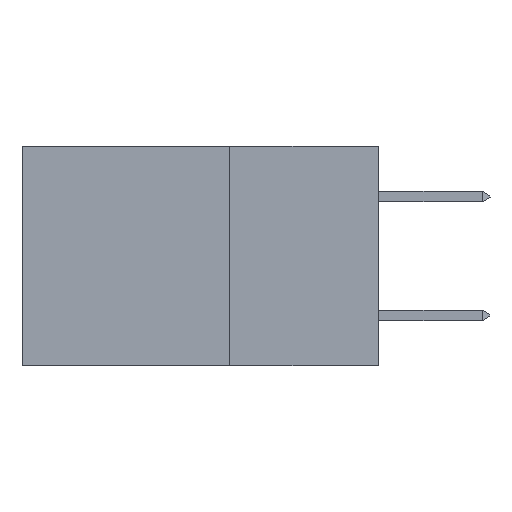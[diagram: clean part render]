
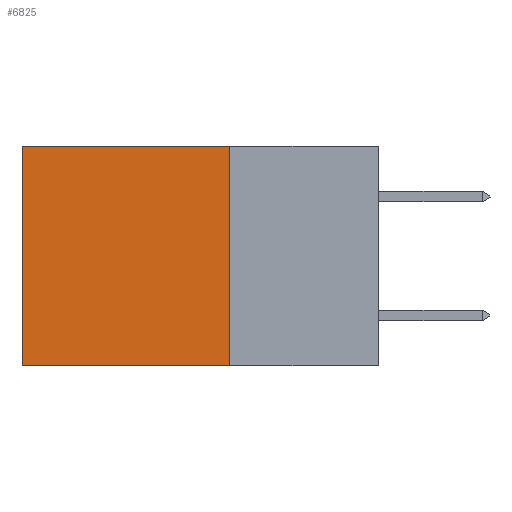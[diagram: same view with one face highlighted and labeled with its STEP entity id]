
A CAD part, left-side view. The second image highlights one B-rep face of the part: STEP entity #6825.
In plain terms, the highlighted planar face has unit normal (-1, 0, 0).
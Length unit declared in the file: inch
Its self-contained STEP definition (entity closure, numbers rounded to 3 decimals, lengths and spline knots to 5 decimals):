
#5 = VERTEX_POINT ( 'NONE', #8557 ) ;
#57 = VECTOR ( 'NONE', #5633, 39.37008 ) ;
#301 = CARTESIAN_POINT ( 'NONE',  ( 0.298, 0.25, -0.37 ) ) ;
#320 = EDGE_CURVE ( 'NONE', #5, #7598, #5847, .T. ) ;
#431 = EDGE_LOOP ( 'NONE', ( #5584, #6023, #5073, #2208 ) ) ;
#1246 = DIRECTION ( 'NONE',  ( 0., 1., 0. ) ) ;
#1287 = EDGE_CURVE ( 'NONE', #1420, #7598, #6776, .T. ) ;
#1373 = AXIS2_PLACEMENT_3D ( 'NONE', #1584, #4476, #4543 ) ;
#1420 = VERTEX_POINT ( 'NONE', #301 ) ;
#1573 = CARTESIAN_POINT ( 'NONE',  ( 0.298, 0.25, -0.37 ) ) ;
#1584 = CARTESIAN_POINT ( 'NONE',  ( 0.298, 0.25, 0. ) ) ;
#1973 = CARTESIAN_POINT ( 'NONE',  ( 0.298, 0.6, 0. ) ) ;
#2208 = ORIENTED_EDGE ( 'NONE', *, *, #9038, .T. ) ;
#2286 = LINE ( 'NONE', #8377, #9173 ) ;
#2630 = LINE ( 'NONE', #6064, #7817 ) ;
#3183 = EDGE_CURVE ( 'NONE', #4567, #1420, #2630, .T. ) ;
#4395 = FACE_OUTER_BOUND ( 'NONE', #431, .T. ) ;
#4476 = DIRECTION ( 'NONE',  ( 1., 0., 0. ) ) ;
#4543 = DIRECTION ( 'NONE',  ( 0., 0., -1. ) ) ;
#4567 = VERTEX_POINT ( 'NONE', #8984 ) ;
#4875 = CARTESIAN_POINT ( 'NONE',  ( 0.298, 0.6, -0.37 ) ) ;
#5073 = ORIENTED_EDGE ( 'NONE', *, *, #3183, .F. ) ;
#5584 = ORIENTED_EDGE ( 'NONE', *, *, #320, .T. ) ;
#5633 = DIRECTION ( 'NONE',  ( 0., 0., -1. ) ) ;
#5847 = LINE ( 'NONE', #1973, #57 ) ;
#6023 = ORIENTED_EDGE ( 'NONE', *, *, #1287, .F. ) ;
#6064 = CARTESIAN_POINT ( 'NONE',  ( 0.298, 0.25, 0. ) ) ;
#6776 = LINE ( 'NONE', #1573, #6995 ) ;
#6825 = ADVANCED_FACE ( 'NONE', ( #4395 ), #8909, .F. ) ;
#6995 = VECTOR ( 'NONE', #8244, 39.37008 ) ;
#7598 = VERTEX_POINT ( 'NONE', #4875 ) ;
#7817 = VECTOR ( 'NONE', #9009, 39.37008 ) ;
#8244 = DIRECTION ( 'NONE',  ( 0., 1., 0. ) ) ;
#8377 = CARTESIAN_POINT ( 'NONE',  ( 0.298, 0.25, 0. ) ) ;
#8557 = CARTESIAN_POINT ( 'NONE',  ( 0.298, 0.6, 0. ) ) ;
#8909 = PLANE ( 'NONE',  #1373 ) ;
#8984 = CARTESIAN_POINT ( 'NONE',  ( 0.298, 0.25, 0. ) ) ;
#9009 = DIRECTION ( 'NONE',  ( 0., 0., -1. ) ) ;
#9038 = EDGE_CURVE ( 'NONE', #4567, #5, #2286, .T. ) ;
#9173 = VECTOR ( 'NONE', #1246, 39.37008 ) ;
